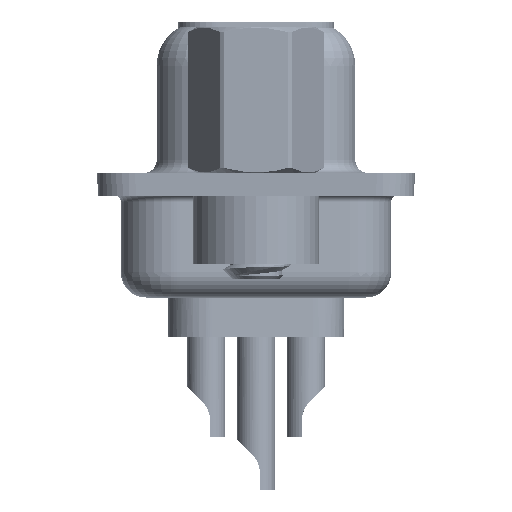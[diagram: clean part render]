
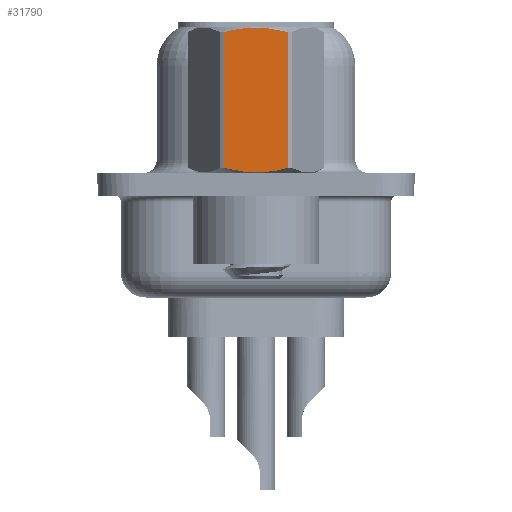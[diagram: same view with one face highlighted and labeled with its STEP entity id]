
A CAD part, left-side view. The second image highlights one B-rep face of the part: STEP entity #31790.
In plain terms, the highlighted planar face has unit normal (-1, 0, 0).
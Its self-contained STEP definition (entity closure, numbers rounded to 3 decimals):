
#1130 = CARTESIAN_POINT ( 'NONE',  ( -2.381, -1.273, 0.652 ) ) ;
#2515 = ORIENTED_EDGE ( 'NONE', *, *, #13881, .T. ) ;
#3218 = B_SPLINE_CURVE_WITH_KNOTS ( 'NONE', 3,
 ( #13413, #25329, #10714, #32422, #17064, #43102, #35589, #17296, #36308, #9754 ),
 .UNSPECIFIED., .F., .F.,
 ( 4, 2, 2, 2, 4 ),
 ( 0.001, 0.002, 0.002, 0.003, 0.004 ),
 .UNSPECIFIED. ) ;
#3493 = CARTESIAN_POINT ( 'NONE',  ( -2.381, 1.273, 0.652 ) ) ;
#4768 = CARTESIAN_POINT ( 'NONE',  ( -2.381, -1.066, 0.596 ) ) ;
#5579 = PLANE ( 'NONE',  #6435 ) ;
#6435 = AXIS2_PLACEMENT_3D ( 'NONE', #31640, #21149, #38945 ) ;
#7041 = CARTESIAN_POINT ( 'NONE',  ( -2.381, 1.273, 3.792 ) ) ;
#7048 = CARTESIAN_POINT ( 'NONE',  ( -2.381, 1.273, 6.048 ) ) ;
#7929 = CARTESIAN_POINT ( 'NONE',  ( -2.381, -0.432, 0.485 ) ) ;
#8732 = EDGE_CURVE ( 'NONE', #21796, #24765, #3218, .T. ) ;
#9400 = VECTOR ( 'NONE', #48075, 1000. ) ;
#9754 = CARTESIAN_POINT ( 'NONE',  ( -2.381, 1.273, 6.048 ) ) ;
#10714 = CARTESIAN_POINT ( 'NONE',  ( -2.381, -0.858, 6.15 ) ) ;
#13337 = LINE ( 'NONE', #28185, #9400 ) ;
#13413 = CARTESIAN_POINT ( 'NONE',  ( -2.381, -1.273, 6.048 ) ) ;
#13881 = EDGE_CURVE ( 'NONE', #24242, #21796, #13337, .T. ) ;
#14859 = B_SPLINE_CURVE_WITH_KNOTS ( 'NONE', 3,
 ( #26197, #23047, #26436, #30102, #37898, #44928, #7929, #23282, #4768, #19604 ),
 .UNSPECIFIED., .F., .F.,
 ( 4, 2, 2, 2, 4 ),
 ( 0.003, 0.003, 0.004, 0.004, 0.005 ),
 .UNSPECIFIED. ) ;
#17064 = CARTESIAN_POINT ( 'NONE',  ( -2.381, -0.215, 6.232 ) ) ;
#17296 = CARTESIAN_POINT ( 'NONE',  ( -2.381, 0.853, 6.151 ) ) ;
#17320 = EDGE_CURVE ( 'NONE', #44517, #24242, #14859, .T. ) ;
#19604 = CARTESIAN_POINT ( 'NONE',  ( -2.381, -1.273, 0.652 ) ) ;
#21149 = DIRECTION ( 'NONE',  ( -1., 0., 0. ) ) ;
#21796 = VERTEX_POINT ( 'NONE', #25379 ) ;
#22541 = ORIENTED_EDGE ( 'NONE', *, *, #46286, .T. ) ;
#23047 = CARTESIAN_POINT ( 'NONE',  ( -2.381, 1.065, 0.596 ) ) ;
#23282 = CARTESIAN_POINT ( 'NONE',  ( -2.381, -0.858, 0.55 ) ) ;
#23864 = FACE_OUTER_BOUND ( 'NONE', #32794, .T. ) ;
#24242 = VERTEX_POINT ( 'NONE', #1130 ) ;
#24765 = VERTEX_POINT ( 'NONE', #7048 ) ;
#25329 = CARTESIAN_POINT ( 'NONE',  ( -2.381, -1.066, 6.104 ) ) ;
#25379 = CARTESIAN_POINT ( 'NONE',  ( -2.381, -1.273, 6.048 ) ) ;
#26197 = CARTESIAN_POINT ( 'NONE',  ( -2.381, 1.273, 0.652 ) ) ;
#26436 = CARTESIAN_POINT ( 'NONE',  ( -2.381, 0.853, 0.549 ) ) ;
#28185 = CARTESIAN_POINT ( 'NONE',  ( -2.381, -1.273, 3.792 ) ) ;
#30102 = CARTESIAN_POINT ( 'NONE',  ( -2.381, 0.428, 0.485 ) ) ;
#31640 = CARTESIAN_POINT ( 'NONE',  ( -2.381, 1.375, -3.75 ) ) ;
#31790 = ADVANCED_FACE ( 'NONE', ( #23864 ), #5579, .T. ) ;
#32422 = CARTESIAN_POINT ( 'NONE',  ( -2.381, -0.432, 6.215 ) ) ;
#32794 = EDGE_LOOP ( 'NONE', ( #47497, #2515, #47603, #22541 ) ) ;
#35589 = CARTESIAN_POINT ( 'NONE',  ( -2.381, 0.428, 6.215 ) ) ;
#35805 = DIRECTION ( 'NONE',  ( 0., 0., -1. ) ) ;
#36308 = CARTESIAN_POINT ( 'NONE',  ( -2.381, 1.065, 6.104 ) ) ;
#37898 = CARTESIAN_POINT ( 'NONE',  ( -2.381, 0.215, 0.468 ) ) ;
#38945 = DIRECTION ( 'NONE',  ( 0., -1., 0. ) ) ;
#40389 = LINE ( 'NONE', #7041, #44806 ) ;
#43102 = CARTESIAN_POINT ( 'NONE',  ( -2.381, 0.215, 6.232 ) ) ;
#44517 = VERTEX_POINT ( 'NONE', #3493 ) ;
#44806 = VECTOR ( 'NONE', #35805, 1000. ) ;
#44928 = CARTESIAN_POINT ( 'NONE',  ( -2.381, -0.215, 0.468 ) ) ;
#46286 = EDGE_CURVE ( 'NONE', #24765, #44517, #40389, .T. ) ;
#47497 = ORIENTED_EDGE ( 'NONE', *, *, #17320, .T. ) ;
#47603 = ORIENTED_EDGE ( 'NONE', *, *, #8732, .T. ) ;
#48075 = DIRECTION ( 'NONE',  ( 0., 0., 1. ) ) ;
